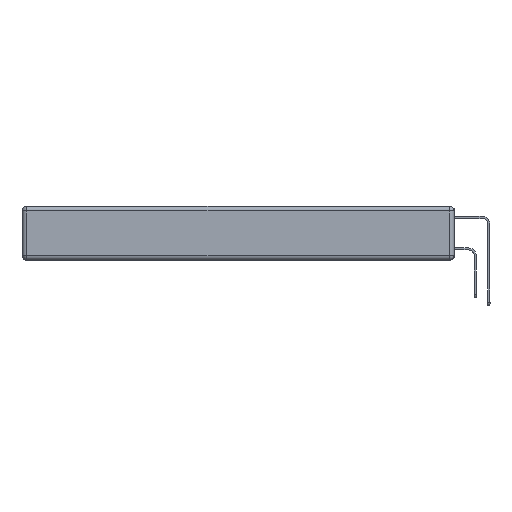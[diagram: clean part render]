
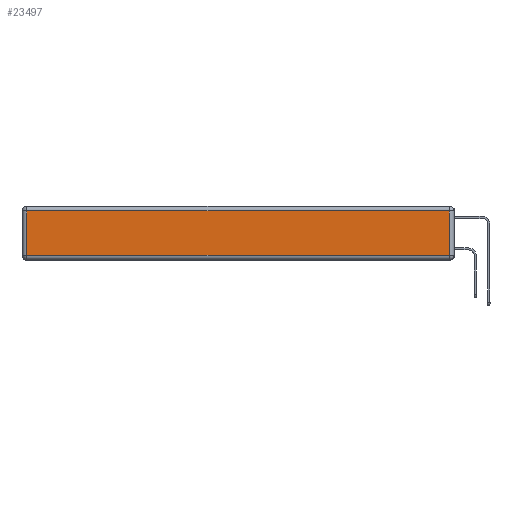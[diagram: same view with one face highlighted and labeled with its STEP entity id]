
A CAD part, left-side view. The second image highlights one B-rep face of the part: STEP entity #23497.
In plain terms, the highlighted planar face has unit normal (-1, 0, 0).
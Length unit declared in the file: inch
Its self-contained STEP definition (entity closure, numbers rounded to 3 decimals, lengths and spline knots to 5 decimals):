
#2694 = CARTESIAN_POINT ( 'NONE',  ( 0., 2.75, -0.03 ) ) ;
#2832 = ORIENTED_EDGE ( 'NONE', *, *, #14204, .T. ) ;
#3374 = LINE ( 'NONE', #17725, #6748 ) ;
#3444 = DIRECTION ( 'NONE',  ( 0., -1., 0. ) ) ;
#3743 = ORIENTED_EDGE ( 'NONE', *, *, #22968, .T. ) ;
#4547 = DIRECTION ( 'NONE',  ( 0., 1., 0. ) ) ;
#6553 = LINE ( 'NONE', #2694, #12686 ) ;
#6748 = VECTOR ( 'NONE', #23322, 39.37008 ) ;
#7034 = LINE ( 'NONE', #23124, #19469 ) ;
#7557 = CARTESIAN_POINT ( 'NONE',  ( 0., 0., -0.313 ) ) ;
#7701 = VERTEX_POINT ( 'NONE', #24552 ) ;
#8828 = CARTESIAN_POINT ( 'NONE',  ( 0., 2.72, -0.03 ) ) ;
#9411 = EDGE_LOOP ( 'NONE', ( #20020, #2832, #22401, #3743 ) ) ;
#12681 = AXIS2_PLACEMENT_3D ( 'NONE', #24511, #14143, #23987 ) ;
#12686 = VECTOR ( 'NONE', #4547, 39.37008 ) ;
#13157 = DIRECTION ( 'NONE',  ( 0., 0., -1. ) ) ;
#14143 = DIRECTION ( 'NONE',  ( -1., 0., 0. ) ) ;
#14204 = EDGE_CURVE ( 'NONE', #7701, #22886, #3374, .T. ) ;
#16401 = PLANE ( 'NONE',  #12681 ) ;
#17725 = CARTESIAN_POINT ( 'NONE',  ( 0., 0.03, -0.343 ) ) ;
#18390 = FACE_OUTER_BOUND ( 'NONE', #9411, .T. ) ;
#19208 = VERTEX_POINT ( 'NONE', #23934 ) ;
#19469 = VECTOR ( 'NONE', #13157, 39.37008 ) ;
#19828 = VERTEX_POINT ( 'NONE', #8828 ) ;
#20020 = ORIENTED_EDGE ( 'NONE', *, *, #23101, .T. ) ;
#21405 = CARTESIAN_POINT ( 'NONE',  ( 0., 0.03, -0.03 ) ) ;
#21671 = LINE ( 'NONE', #7557, #22916 ) ;
#22205 = EDGE_CURVE ( 'NONE', #22886, #19828, #6553, .T. ) ;
#22401 = ORIENTED_EDGE ( 'NONE', *, *, #22205, .T. ) ;
#22886 = VERTEX_POINT ( 'NONE', #21405 ) ;
#22916 = VECTOR ( 'NONE', #3444, 39.37008 ) ;
#22968 = EDGE_CURVE ( 'NONE', #19828, #19208, #7034, .T. ) ;
#23101 = EDGE_CURVE ( 'NONE', #19208, #7701, #21671, .T. ) ;
#23124 = CARTESIAN_POINT ( 'NONE',  ( 0., 2.72, -0.343 ) ) ;
#23322 = DIRECTION ( 'NONE',  ( 0., 0., 1. ) ) ;
#23497 = ADVANCED_FACE ( 'NONE', ( #18390 ), #16401, .T. ) ;
#23934 = CARTESIAN_POINT ( 'NONE',  ( 0., 2.72, -0.313 ) ) ;
#23987 = DIRECTION ( 'NONE',  ( 0., 0., 1. ) ) ;
#24511 = CARTESIAN_POINT ( 'NONE',  ( 0., 0., -0.343 ) ) ;
#24552 = CARTESIAN_POINT ( 'NONE',  ( 0., 0.03, -0.313 ) ) ;
